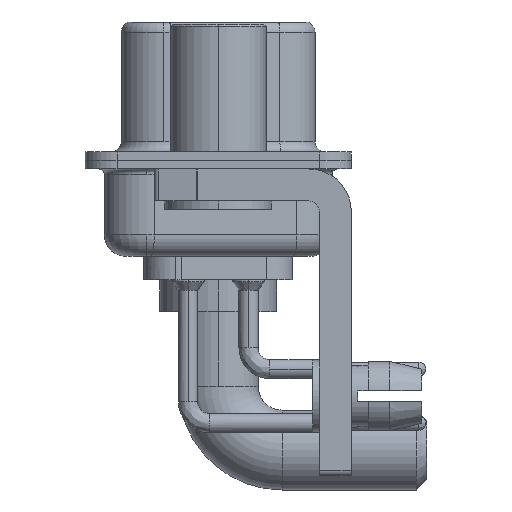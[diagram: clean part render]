
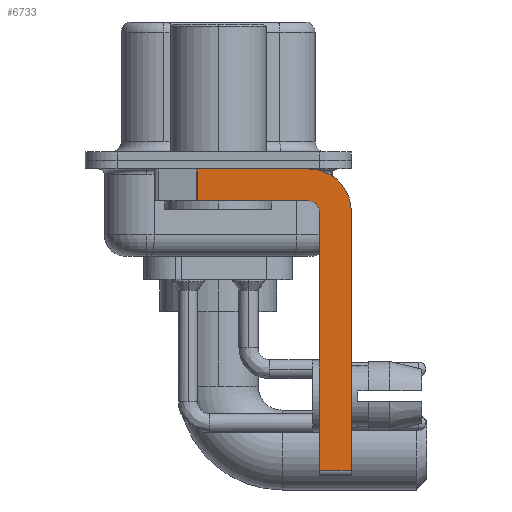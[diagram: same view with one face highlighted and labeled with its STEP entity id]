
A CAD part, left-side view. The second image highlights one B-rep face of the part: STEP entity #6733.
In plain terms, the highlighted planar face has unit normal (-1, 0, 0).
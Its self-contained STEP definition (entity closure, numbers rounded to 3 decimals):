
#131 = CIRCLE ( 'NONE', #11287, 0.5 ) ;
#333 = ORIENTED_EDGE ( 'NONE', *, *, #9871, .F. ) ;
#339 = CARTESIAN_POINT ( 'NONE',  ( -2.9, 0.978, -1.9 ) ) ;
#751 = LINE ( 'NONE', #24271, #27577 ) ;
#958 = EDGE_CURVE ( 'NONE', #22283, #28530, #751, .T. ) ;
#1078 = DIRECTION ( 'NONE',  ( 0., 0., -1. ) ) ;
#1871 = ORIENTED_EDGE ( 'NONE', *, *, #28138, .T. ) ;
#2010 = VERTEX_POINT ( 'NONE', #11234 ) ;
#2830 = VERTEX_POINT ( 'NONE', #10706 ) ;
#2860 = DIRECTION ( 'NONE',  ( -1., 0., 0. ) ) ;
#3022 = DIRECTION ( 'NONE',  ( 0., -1., 0. ) ) ;
#3092 = CARTESIAN_POINT ( 'NONE',  ( -2.9, -4.25, -2.4 ) ) ;
#3821 = CARTESIAN_POINT ( 'NONE',  ( -2.9, -6.25, -2.4 ) ) ;
#4040 = VECTOR ( 'NONE', #20882, 1000. ) ;
#4652 = LINE ( 'NONE', #23051, #26343 ) ;
#5313 = VERTEX_POINT ( 'NONE', #26728 ) ;
#5783 = DIRECTION ( 'NONE',  ( 0., 0., -1. ) ) ;
#6379 = VERTEX_POINT ( 'NONE', #10993 ) ;
#6733 = ADVANCED_FACE ( 'NONE', ( #12193 ), #7327, .F. ) ;
#7269 = CARTESIAN_POINT ( 'NONE',  ( -2.9, -6.25, -14.55 ) ) ;
#7327 = PLANE ( 'NONE',  #16489 ) ;
#7866 = DIRECTION ( 'NONE',  ( 0., 0., 1. ) ) ;
#8014 = DIRECTION ( 'NONE',  ( 0., 0., 1. ) ) ;
#8381 = LINE ( 'NONE', #3821, #13304 ) ;
#8608 = AXIS2_PLACEMENT_3D ( 'NONE', #21720, #28255, #1078 ) ;
#8675 = VERTEX_POINT ( 'NONE', #20926 ) ;
#9128 = EDGE_CURVE ( 'NONE', #8675, #5313, #25458, .T. ) ;
#9480 = ORIENTED_EDGE ( 'NONE', *, *, #9128, .F. ) ;
#9851 = CARTESIAN_POINT ( 'NONE',  ( -2.9, -4.25, -2.4 ) ) ;
#9871 = EDGE_CURVE ( 'NONE', #19431, #28530, #8381, .T. ) ;
#10009 = ORIENTED_EDGE ( 'NONE', *, *, #14588, .F. ) ;
#10202 = DIRECTION ( 'NONE',  ( 1., 0., 0. ) ) ;
#10706 = CARTESIAN_POINT ( 'NONE',  ( -2.9, 0.978, -0.4 ) ) ;
#10928 = CARTESIAN_POINT ( 'NONE',  ( -2.9, -6.25, -2.4 ) ) ;
#10993 = CARTESIAN_POINT ( 'NONE',  ( -2.9, -4.75, -2.4 ) ) ;
#11221 = CARTESIAN_POINT ( 'NONE',  ( -2.9, -4.75, -14.55 ) ) ;
#11234 = CARTESIAN_POINT ( 'NONE',  ( -2.9, -4.25, -0.4 ) ) ;
#11287 = AXIS2_PLACEMENT_3D ( 'NONE', #9851, #2860, #8014 ) ;
#11468 = CARTESIAN_POINT ( 'NONE',  ( -2.9, -4.25, -1.9 ) ) ;
#11625 = DIRECTION ( 'NONE',  ( 0., -1., 0. ) ) ;
#11669 = VECTOR ( 'NONE', #7866, 1000. ) ;
#12193 = FACE_OUTER_BOUND ( 'NONE', #23349, .T. ) ;
#12284 = LINE ( 'NONE', #28669, #11669 ) ;
#13206 = EDGE_CURVE ( 'NONE', #6379, #8675, #131, .T. ) ;
#13304 = VECTOR ( 'NONE', #5783, 1000. ) ;
#13649 = VECTOR ( 'NONE', #18871, 1000. ) ;
#14588 = EDGE_CURVE ( 'NONE', #22283, #6379, #12284, .T. ) ;
#16489 = AXIS2_PLACEMENT_3D ( 'NONE', #3092, #10202, #26163 ) ;
#17479 = ORIENTED_EDGE ( 'NONE', *, *, #13206, .F. ) ;
#18871 = DIRECTION ( 'NONE',  ( 0., 0., -1. ) ) ;
#19262 = ORIENTED_EDGE ( 'NONE', *, *, #19294, .F. ) ;
#19294 = EDGE_CURVE ( 'NONE', #2010, #19431, #26093, .T. ) ;
#19431 = VERTEX_POINT ( 'NONE', #10928 ) ;
#20882 = DIRECTION ( 'NONE',  ( 0., 1., 0. ) ) ;
#20926 = CARTESIAN_POINT ( 'NONE',  ( -2.9, -4.25, -1.9 ) ) ;
#21720 = CARTESIAN_POINT ( 'NONE',  ( -2.9, -4.25, -2.4 ) ) ;
#22283 = VERTEX_POINT ( 'NONE', #11221 ) ;
#22944 = EDGE_CURVE ( 'NONE', #2830, #2010, #4652, .T. ) ;
#23051 = CARTESIAN_POINT ( 'NONE',  ( -2.9, 3., -0.4 ) ) ;
#23349 = EDGE_LOOP ( 'NONE', ( #29214, #1871, #9480, #17479, #10009, #28950, #333, #19262 ) ) ;
#23444 = LINE ( 'NONE', #339, #13649 ) ;
#24271 = CARTESIAN_POINT ( 'NONE',  ( -2.9, -4.25, -14.55 ) ) ;
#25458 = LINE ( 'NONE', #11468, #4040 ) ;
#26093 = CIRCLE ( 'NONE', #8608, 2. ) ;
#26163 = DIRECTION ( 'NONE',  ( 0., 0., -1. ) ) ;
#26343 = VECTOR ( 'NONE', #11625, 1000. ) ;
#26728 = CARTESIAN_POINT ( 'NONE',  ( -2.9, 0.978, -1.9 ) ) ;
#27577 = VECTOR ( 'NONE', #3022, 1000. ) ;
#28138 = EDGE_CURVE ( 'NONE', #2830, #5313, #23444, .T. ) ;
#28255 = DIRECTION ( 'NONE',  ( 1., 0., 0. ) ) ;
#28530 = VERTEX_POINT ( 'NONE', #7269 ) ;
#28669 = CARTESIAN_POINT ( 'NONE',  ( -2.9, -4.75, -14.8 ) ) ;
#28950 = ORIENTED_EDGE ( 'NONE', *, *, #958, .T. ) ;
#29214 = ORIENTED_EDGE ( 'NONE', *, *, #22944, .F. ) ;
